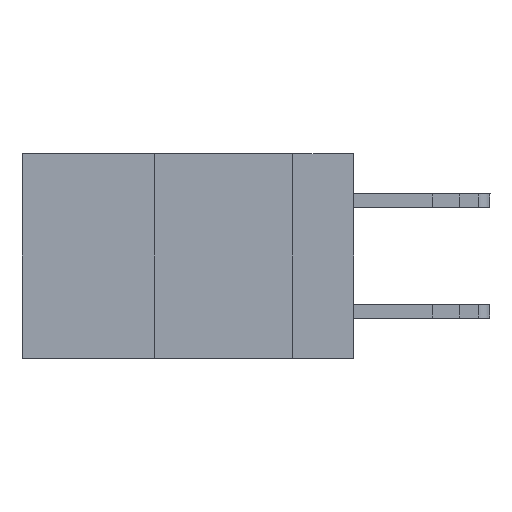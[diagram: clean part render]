
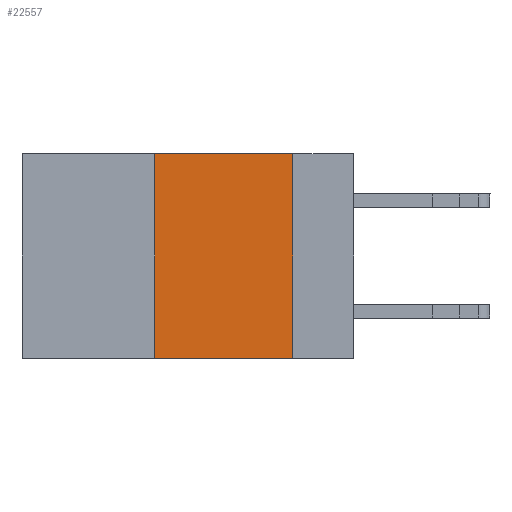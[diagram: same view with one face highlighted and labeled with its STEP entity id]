
A CAD part, left-side view. The second image highlights one B-rep face of the part: STEP entity #22557.
In plain terms, the highlighted planar face has unit normal (-1, 0, 0).
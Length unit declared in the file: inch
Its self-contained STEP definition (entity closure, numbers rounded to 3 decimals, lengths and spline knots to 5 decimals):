
#1892 = ORIENTED_EDGE ( 'NONE', *, *, #21137, .F. ) ;
#3295 = ORIENTED_EDGE ( 'NONE', *, *, #20797, .T. ) ;
#4133 = CARTESIAN_POINT ( 'NONE',  ( 0., 0.11, -0.37 ) ) ;
#4822 = CARTESIAN_POINT ( 'NONE',  ( 0., 0.36, 0. ) ) ;
#5060 = VECTOR ( 'NONE', #34002, 39.37008 ) ;
#6679 = AXIS2_PLACEMENT_3D ( 'NONE', #13285, #38126, #25560 ) ;
#6914 = LINE ( 'NONE', #22213, #5060 ) ;
#7196 = DIRECTION ( 'NONE',  ( 0., 0., -1. ) ) ;
#9901 = CARTESIAN_POINT ( 'NONE',  ( 0., 0.36, 0. ) ) ;
#10380 = VERTEX_POINT ( 'NONE', #16729 ) ;
#11194 = LINE ( 'NONE', #34193, #16388 ) ;
#13193 = VECTOR ( 'NONE', #31619, 39.37008 ) ;
#13285 = CARTESIAN_POINT ( 'NONE',  ( 0., 0.6, 0. ) ) ;
#15427 = LINE ( 'NONE', #9901, #16895 ) ;
#16388 = VECTOR ( 'NONE', #7196, 39.37008 ) ;
#16729 = CARTESIAN_POINT ( 'NONE',  ( 0., 0.11, 0. ) ) ;
#16895 = VECTOR ( 'NONE', #21760, 39.37008 ) ;
#18312 = VERTEX_POINT ( 'NONE', #4822 ) ;
#19989 = VERTEX_POINT ( 'NONE', #4133 ) ;
#20797 = EDGE_CURVE ( 'NONE', #38143, #19989, #39518, .T. ) ;
#21137 = EDGE_CURVE ( 'NONE', #18312, #10380, #6914, .T. ) ;
#21302 = EDGE_LOOP ( 'NONE', ( #25777, #1892, #31630, #3295 ) ) ;
#21760 = DIRECTION ( 'NONE',  ( 0., 0., 1. ) ) ;
#21818 = EDGE_CURVE ( 'NONE', #38143, #18312, #15427, .T. ) ;
#21820 = EDGE_CURVE ( 'NONE', #10380, #19989, #11194, .T. ) ;
#22213 = CARTESIAN_POINT ( 'NONE',  ( 0., 0.6, 0. ) ) ;
#22557 = ADVANCED_FACE ( 'NONE', ( #23053 ), #34779, .F. ) ;
#23053 = FACE_OUTER_BOUND ( 'NONE', #21302, .T. ) ;
#25560 = DIRECTION ( 'NONE',  ( 0., 0., -1. ) ) ;
#25777 = ORIENTED_EDGE ( 'NONE', *, *, #21820, .F. ) ;
#30251 = CARTESIAN_POINT ( 'NONE',  ( 0., 0.36, -0.37 ) ) ;
#31619 = DIRECTION ( 'NONE',  ( 0., -1., 0. ) ) ;
#31630 = ORIENTED_EDGE ( 'NONE', *, *, #21818, .F. ) ;
#34002 = DIRECTION ( 'NONE',  ( 0., -1., 0. ) ) ;
#34193 = CARTESIAN_POINT ( 'NONE',  ( 0., 0.11, 0. ) ) ;
#34779 = PLANE ( 'NONE',  #6679 ) ;
#35078 = CARTESIAN_POINT ( 'NONE',  ( 0., 0.6, -0.37 ) ) ;
#38126 = DIRECTION ( 'NONE',  ( 1., 0., 0. ) ) ;
#38143 = VERTEX_POINT ( 'NONE', #30251 ) ;
#39518 = LINE ( 'NONE', #35078, #13193 ) ;
